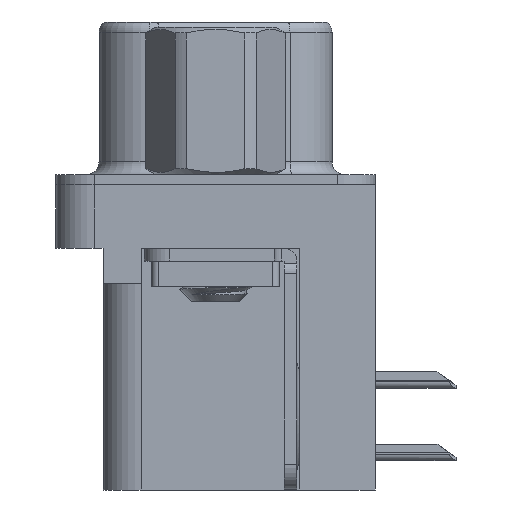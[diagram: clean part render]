
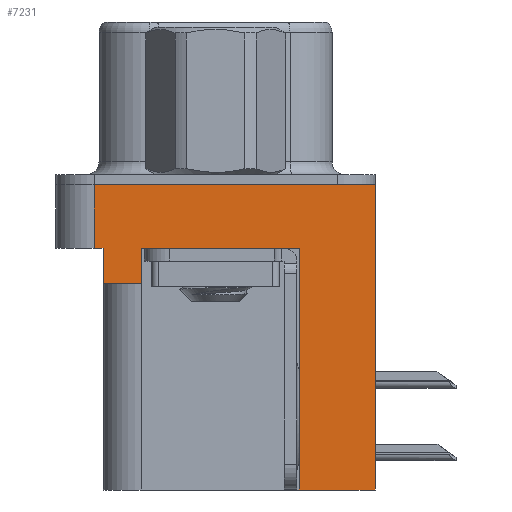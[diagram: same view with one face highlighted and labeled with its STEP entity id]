
A CAD part, left-side view. The second image highlights one B-rep face of the part: STEP entity #7231.
In plain terms, the highlighted planar face has unit normal (-1, 0, 0).
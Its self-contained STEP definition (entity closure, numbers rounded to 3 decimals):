
#206 = VECTOR ( 'NONE', #16558, 1000. ) ;
#446 = ORIENTED_EDGE ( 'NONE', *, *, #20556, .T. ) ;
#484 = ORIENTED_EDGE ( 'NONE', *, *, #26984, .F. ) ;
#606 = LINE ( 'NONE', #17009, #26694 ) ;
#1200 = LINE ( 'NONE', #27501, #3626 ) ;
#1542 = VERTEX_POINT ( 'NONE', #32836 ) ;
#1709 = EDGE_CURVE ( 'NONE', #1542, #32740, #1200, .T. ) ;
#3214 = CARTESIAN_POINT ( 'NONE',  ( -2.91, -6.275, -2.5 ) ) ;
#3551 = DIRECTION ( 'NONE',  ( 0., -1., 0. ) ) ;
#3626 = VECTOR ( 'NONE', #3551, 1000. ) ;
#4908 = VECTOR ( 'NONE', #5840, 1000. ) ;
#4973 = EDGE_CURVE ( 'NONE', #11062, #10084, #11006, .T. ) ;
#5278 = VERTEX_POINT ( 'NONE', #18557 ) ;
#5784 = CARTESIAN_POINT ( 'NONE',  ( -2.91, 4.775, 0. ) ) ;
#5840 = DIRECTION ( 'NONE',  ( 0., -1., 0. ) ) ;
#6322 = ORIENTED_EDGE ( 'NONE', *, *, #17135, .F. ) ;
#6480 = CARTESIAN_POINT ( 'NONE',  ( -2.91, -3.295, -12. ) ) ;
#6755 = CARTESIAN_POINT ( 'NONE',  ( -2.91, -6.275, -12. ) ) ;
#7073 = DIRECTION ( 'NONE',  ( 0., 1., 0. ) ) ;
#7231 = ADVANCED_FACE ( 'NONE', ( #29544 ), #30092, .T. ) ;
#7682 = ORIENTED_EDGE ( 'NONE', *, *, #1709, .T. ) ;
#7823 = AXIS2_PLACEMENT_3D ( 'NONE', #29854, #19414, #9093 ) ;
#8327 = LINE ( 'NONE', #24984, #23913 ) ;
#8565 = DIRECTION ( 'NONE',  ( 0., 0., 1. ) ) ;
#8752 = VECTOR ( 'NONE', #21919, 1000. ) ;
#8756 = EDGE_LOOP ( 'NONE', ( #15681, #6322, #446, #15650, #26986, #28402, #7682, #18599, #484, #17353 ) ) ;
#9093 = DIRECTION ( 'NONE',  ( 0., 0., 1. ) ) ;
#9310 = DIRECTION ( 'NONE',  ( 0., 1., 0. ) ) ;
#10084 = VERTEX_POINT ( 'NONE', #29098 ) ;
#11006 = LINE ( 'NONE', #28350, #33468 ) ;
#11062 = VERTEX_POINT ( 'NONE', #19425 ) ;
#11176 = EDGE_CURVE ( 'NONE', #13681, #14583, #28915, .T. ) ;
#11192 = CARTESIAN_POINT ( 'NONE',  ( -2.91, -3.295, -12. ) ) ;
#11532 = VERTEX_POINT ( 'NONE', #6480 ) ;
#13046 = LINE ( 'NONE', #3214, #4908 ) ;
#13681 = VERTEX_POINT ( 'NONE', #5784 ) ;
#14084 = LINE ( 'NONE', #16672, #206 ) ;
#14412 = EDGE_CURVE ( 'NONE', #10084, #14732, #15420, .T. ) ;
#14583 = VERTEX_POINT ( 'NONE', #21032 ) ;
#14732 = VERTEX_POINT ( 'NONE', #23667 ) ;
#15268 = DIRECTION ( 'NONE',  ( 0., -1., 0. ) ) ;
#15420 = LINE ( 'NONE', #24254, #33782 ) ;
#15650 = ORIENTED_EDGE ( 'NONE', *, *, #14412, .F. ) ;
#15681 = ORIENTED_EDGE ( 'NONE', *, *, #11176, .F. ) ;
#16558 = DIRECTION ( 'NONE',  ( 0., 0., 1. ) ) ;
#16672 = CARTESIAN_POINT ( 'NONE',  ( -2.91, 4.775, -2.5 ) ) ;
#16985 = VECTOR ( 'NONE', #29435, 1000. ) ;
#17009 = CARTESIAN_POINT ( 'NONE',  ( -2.91, 2.895, -3.9 ) ) ;
#17135 = EDGE_CURVE ( 'NONE', #5278, #13681, #14084, .T. ) ;
#17353 = ORIENTED_EDGE ( 'NONE', *, *, #31181, .T. ) ;
#18557 = CARTESIAN_POINT ( 'NONE',  ( -2.91, 4.775, -2.5 ) ) ;
#18599 = ORIENTED_EDGE ( 'NONE', *, *, #30838, .F. ) ;
#19414 = DIRECTION ( 'NONE',  ( -1., 0., 0. ) ) ;
#19425 = CARTESIAN_POINT ( 'NONE',  ( -2.91, 2.895, -3.9 ) ) ;
#20411 = CARTESIAN_POINT ( 'NONE',  ( -2.91, -6.275, 0. ) ) ;
#20556 = EDGE_CURVE ( 'NONE', #5278, #14732, #13046, .T. ) ;
#21032 = CARTESIAN_POINT ( 'NONE',  ( -2.91, -6.275, 0. ) ) ;
#21919 = DIRECTION ( 'NONE',  ( 0., 0., 1. ) ) ;
#23667 = CARTESIAN_POINT ( 'NONE',  ( -2.91, 4.425, -2.5 ) ) ;
#23913 = VECTOR ( 'NONE', #9310, 1000. ) ;
#23941 = LINE ( 'NONE', #11192, #16985 ) ;
#24254 = CARTESIAN_POINT ( 'NONE',  ( -2.91, 4.425, -3.9 ) ) ;
#24681 = VERTEX_POINT ( 'NONE', #6755 ) ;
#24766 = CARTESIAN_POINT ( 'NONE',  ( -2.91, -6.275, -2.5 ) ) ;
#24984 = CARTESIAN_POINT ( 'NONE',  ( -2.91, -3.295, -12. ) ) ;
#26694 = VECTOR ( 'NONE', #30074, 1000. ) ;
#26984 = EDGE_CURVE ( 'NONE', #24681, #11532, #8327, .T. ) ;
#26986 = ORIENTED_EDGE ( 'NONE', *, *, #4973, .F. ) ;
#27501 = CARTESIAN_POINT ( 'NONE',  ( -2.91, -6.275, -2.5 ) ) ;
#28350 = CARTESIAN_POINT ( 'NONE',  ( -2.91, 4.425, -3.9 ) ) ;
#28402 = ORIENTED_EDGE ( 'NONE', *, *, #31275, .T. ) ;
#28915 = LINE ( 'NONE', #20411, #30534 ) ;
#29098 = CARTESIAN_POINT ( 'NONE',  ( -2.91, 4.425, -3.9 ) ) ;
#29435 = DIRECTION ( 'NONE',  ( 0., 0., 1. ) ) ;
#29544 = FACE_OUTER_BOUND ( 'NONE', #8756, .T. ) ;
#29854 = CARTESIAN_POINT ( 'NONE',  ( -2.91, -6.275, -2.5 ) ) ;
#30074 = DIRECTION ( 'NONE',  ( 0., 0., 1. ) ) ;
#30092 = PLANE ( 'NONE',  #7823 ) ;
#30534 = VECTOR ( 'NONE', #15268, 1000. ) ;
#30838 = EDGE_CURVE ( 'NONE', #11532, #32740, #23941, .T. ) ;
#31181 = EDGE_CURVE ( 'NONE', #24681, #14583, #33641, .T. ) ;
#31275 = EDGE_CURVE ( 'NONE', #11062, #1542, #606, .T. ) ;
#32381 = CARTESIAN_POINT ( 'NONE',  ( -2.91, -3.295, -2.5 ) ) ;
#32740 = VERTEX_POINT ( 'NONE', #32381 ) ;
#32836 = CARTESIAN_POINT ( 'NONE',  ( -2.91, 2.895, -2.5 ) ) ;
#33468 = VECTOR ( 'NONE', #7073, 1000. ) ;
#33641 = LINE ( 'NONE', #24766, #8752 ) ;
#33782 = VECTOR ( 'NONE', #8565, 1000. ) ;
